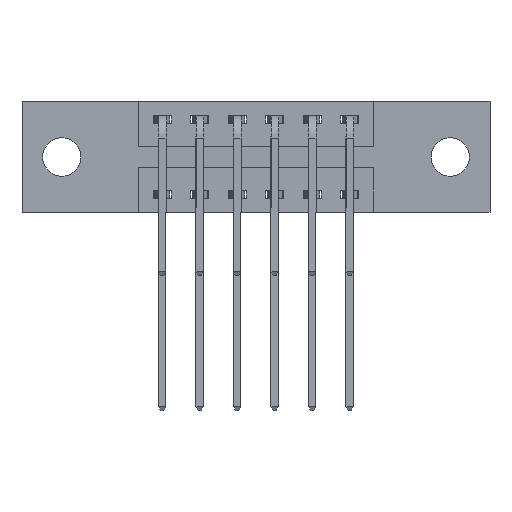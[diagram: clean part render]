
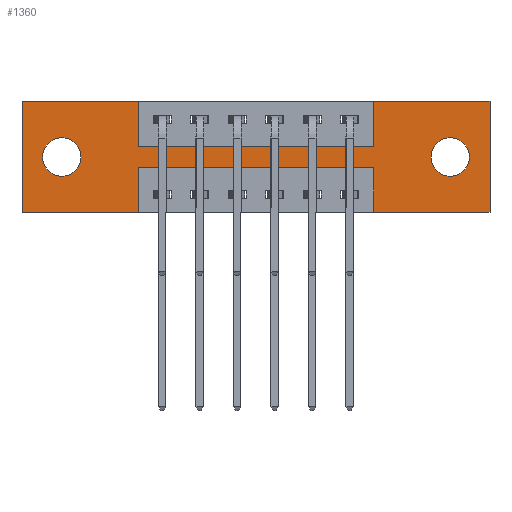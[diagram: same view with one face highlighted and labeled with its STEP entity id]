
A CAD part, front view. The second image highlights one B-rep face of the part: STEP entity #1360.
In plain terms, the highlighted planar face has unit normal (0, -1, 0).
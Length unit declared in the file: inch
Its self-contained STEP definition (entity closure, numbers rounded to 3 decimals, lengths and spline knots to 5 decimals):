
#8 = CARTESIAN_POINT ( 'NONE',  ( 1.56, 0., 0. ) ) ;
#78 = CARTESIAN_POINT ( 'NONE',  ( 0., 0., 0. ) ) ;
#110 = CARTESIAN_POINT ( 'NONE',  ( 0.3875, 0., -0.15 ) ) ;
#120 = LINE ( 'NONE', #2694, #4599 ) ;
#179 = CARTESIAN_POINT ( 'NONE',  ( 0.3875, 0., 0. ) ) ;
#503 = CARTESIAN_POINT ( 'NONE',  ( 0., 0., -0.37 ) ) ;
#523 = ORIENTED_EDGE ( 'NONE', *, *, #1006, .T. ) ;
#839 = DIRECTION ( 'NONE',  ( 0., 0., 1. ) ) ;
#906 = DIRECTION ( 'NONE',  ( 1., 0., 0. ) ) ;
#909 = EDGE_LOOP ( 'NONE', ( #4469, #9878 ) ) ;
#922 = VERTEX_POINT ( 'NONE', #8142 ) ;
#1006 = EDGE_CURVE ( 'NONE', #922, #10519, #6691, .T. ) ;
#1049 = LINE ( 'NONE', #110, #5203 ) ;
#1198 = EDGE_CURVE ( 'NONE', #1411, #8099, #6071, .T. ) ;
#1360 = ADVANCED_FACE ( 'NONE', ( #3206, #5055, #7134 ), #6268, .T. ) ;
#1411 = VERTEX_POINT ( 'NONE', #6201 ) ;
#1429 = DIRECTION ( 'NONE',  ( -1., 0., 0. ) ) ;
#1468 = DIRECTION ( 'NONE',  ( 1., 0., 0. ) ) ;
#1598 = EDGE_LOOP ( 'NONE', ( #10028, #1621, #8962, #8791, #6315, #3848, #6308, #6206, #7337, #6058, #9000, #7433 ) ) ;
#1621 = ORIENTED_EDGE ( 'NONE', *, *, #5158, .F. ) ;
#1800 = VERTEX_POINT ( 'NONE', #5182 ) ;
#1853 = LINE ( 'NONE', #2755, #8150 ) ;
#1967 = CARTESIAN_POINT ( 'NONE',  ( 1.1725, 0., 0. ) ) ;
#2053 = DIRECTION ( 'NONE',  ( 0., 1., 0. ) ) ;
#2152 = VECTOR ( 'NONE', #1429, 39.37008 ) ;
#2493 = CARTESIAN_POINT ( 'NONE',  ( 1.4275, 0., -0.249 ) ) ;
#2647 = CARTESIAN_POINT ( 'NONE',  ( 1.4275, 0., -0.185 ) ) ;
#2694 = CARTESIAN_POINT ( 'NONE',  ( 0.3875, 0., -0.37 ) ) ;
#2755 = CARTESIAN_POINT ( 'NONE',  ( 0., 0., 0. ) ) ;
#3206 = FACE_BOUND ( 'NONE', #909, .T. ) ;
#3214 = EDGE_LOOP ( 'NONE', ( #9630, #523 ) ) ;
#3297 = AXIS2_PLACEMENT_3D ( 'NONE', #7207, #4465, #5010 ) ;
#3348 = LINE ( 'NONE', #1967, #7286 ) ;
#3433 = CARTESIAN_POINT ( 'NONE',  ( 0., 0., -0.37 ) ) ;
#3558 = DIRECTION ( 'NONE',  ( 0., 0., -1. ) ) ;
#3589 = VECTOR ( 'NONE', #5316, 39.37008 ) ;
#3848 = ORIENTED_EDGE ( 'NONE', *, *, #1198, .F. ) ;
#4050 = VERTEX_POINT ( 'NONE', #2493 ) ;
#4059 = VERTEX_POINT ( 'NONE', #3433 ) ;
#4079 = LINE ( 'NONE', #7612, #10232 ) ;
#4196 = VERTEX_POINT ( 'NONE', #7452 ) ;
#4286 = EDGE_CURVE ( 'NONE', #4059, #4196, #1853, .T. ) ;
#4334 = LINE ( 'NONE', #9366, #6192 ) ;
#4375 = EDGE_CURVE ( 'NONE', #8099, #6801, #7669, .T. ) ;
#4419 = DIRECTION ( 'NONE',  ( 0., 0., 1. ) ) ;
#4465 = DIRECTION ( 'NONE',  ( 0., 1., 0. ) ) ;
#4469 = ORIENTED_EDGE ( 'NONE', *, *, #4899, .T. ) ;
#4475 = EDGE_CURVE ( 'NONE', #4050, #8294, #6928, .T. ) ;
#4529 = CARTESIAN_POINT ( 'NONE',  ( 0.3875, 0., -0.22 ) ) ;
#4531 = EDGE_CURVE ( 'NONE', #6801, #1800, #4334, .T. ) ;
#4570 = DIRECTION ( 'NONE',  ( 0., 0., 1. ) ) ;
#4599 = VECTOR ( 'NONE', #5973, 39.37008 ) ;
#4742 = EDGE_CURVE ( 'NONE', #8992, #4059, #8492, .T. ) ;
#4782 = LINE ( 'NONE', #78, #8660 ) ;
#4784 = DIRECTION ( 'NONE',  ( 0., 0., -1. ) ) ;
#4899 = EDGE_CURVE ( 'NONE', #8294, #4050, #5324, .T. ) ;
#4996 = EDGE_CURVE ( 'NONE', #8568, #8992, #120, .T. ) ;
#5010 = DIRECTION ( 'NONE',  ( 0., 0., 1. ) ) ;
#5011 = AXIS2_PLACEMENT_3D ( 'NONE', #2647, #8249, #3558 ) ;
#5014 = EDGE_CURVE ( 'NONE', #10519, #922, #6427, .T. ) ;
#5055 = FACE_BOUND ( 'NONE', #3214, .T. ) ;
#5075 = EDGE_CURVE ( 'NONE', #1800, #9002, #4079, .T. ) ;
#5158 = EDGE_CURVE ( 'NONE', #9002, #8568, #8027, .T. ) ;
#5182 = CARTESIAN_POINT ( 'NONE',  ( 1.1725, 0., -0.37 ) ) ;
#5191 = EDGE_CURVE ( 'NONE', #6055, #8552, #1049, .T. ) ;
#5193 = EDGE_CURVE ( 'NONE', #8552, #1411, #3348, .T. ) ;
#5203 = VECTOR ( 'NONE', #6924, 39.37008 ) ;
#5217 = CARTESIAN_POINT ( 'NONE',  ( 0.1325, 0., -0.185 ) ) ;
#5219 = CARTESIAN_POINT ( 'NONE',  ( 1.1725, 0., -0.22 ) ) ;
#5316 = DIRECTION ( 'NONE',  ( -1., 0., 0. ) ) ;
#5322 = EDGE_CURVE ( 'NONE', #9239, #6055, #8357, .T. ) ;
#5323 = DIRECTION ( 'NONE',  ( 0., 0., -1. ) ) ;
#5324 = CIRCLE ( 'NONE', #5011, 0.064 ) ;
#5590 = VECTOR ( 'NONE', #5323, 39.37008 ) ;
#5720 = CARTESIAN_POINT ( 'NONE',  ( 0.1325, 0., -0.121 ) ) ;
#5768 = CARTESIAN_POINT ( 'NONE',  ( 0.3875, 0., -0.22 ) ) ;
#5826 = VECTOR ( 'NONE', #1468, 39.37008 ) ;
#5973 = DIRECTION ( 'NONE',  ( 0., 0., -1. ) ) ;
#6006 = DIRECTION ( 'NONE',  ( 0., 0., 1. ) ) ;
#6055 = VERTEX_POINT ( 'NONE', #6158 ) ;
#6056 = AXIS2_PLACEMENT_3D ( 'NONE', #5217, #10553, #6006 ) ;
#6058 = ORIENTED_EDGE ( 'NONE', *, *, #9107, .F. ) ;
#6071 = LINE ( 'NONE', #10139, #5826 ) ;
#6158 = CARTESIAN_POINT ( 'NONE',  ( 0.3875, 0., -0.15 ) ) ;
#6192 = VECTOR ( 'NONE', #10109, 39.37008 ) ;
#6201 = CARTESIAN_POINT ( 'NONE',  ( 1.1725, 0., 0. ) ) ;
#6206 = ORIENTED_EDGE ( 'NONE', *, *, #5191, .F. ) ;
#6268 = PLANE ( 'NONE',  #10288 ) ;
#6308 = ORIENTED_EDGE ( 'NONE', *, *, #5193, .F. ) ;
#6315 = ORIENTED_EDGE ( 'NONE', *, *, #4375, .F. ) ;
#6427 = CIRCLE ( 'NONE', #6056, 0.064 ) ;
#6691 = CIRCLE ( 'NONE', #3297, 0.064 ) ;
#6801 = VERTEX_POINT ( 'NONE', #8296 ) ;
#6924 = DIRECTION ( 'NONE',  ( 1., 0., 0. ) ) ;
#6928 = CIRCLE ( 'NONE', #8830, 0.064 ) ;
#6998 = CARTESIAN_POINT ( 'NONE',  ( 1.4275, 0., -0.185 ) ) ;
#7134 = FACE_OUTER_BOUND ( 'NONE', #1598, .T. ) ;
#7207 = CARTESIAN_POINT ( 'NONE',  ( 0.1325, 0., -0.185 ) ) ;
#7286 = VECTOR ( 'NONE', #4570, 39.37008 ) ;
#7337 = ORIENTED_EDGE ( 'NONE', *, *, #5322, .F. ) ;
#7342 = CARTESIAN_POINT ( 'NONE',  ( 0., 0., -0.37 ) ) ;
#7433 = ORIENTED_EDGE ( 'NONE', *, *, #4742, .F. ) ;
#7452 = CARTESIAN_POINT ( 'NONE',  ( 0., 0., 0. ) ) ;
#7612 = CARTESIAN_POINT ( 'NONE',  ( 1.1725, 0., -0.37 ) ) ;
#7669 = LINE ( 'NONE', #8, #5590 ) ;
#7788 = DIRECTION ( 'NONE',  ( 0., 0., -1. ) ) ;
#7800 = DIRECTION ( 'NONE',  ( 0., 0., -1. ) ) ;
#7801 = CARTESIAN_POINT ( 'NONE',  ( 1.56, 0., 0. ) ) ;
#8027 = LINE ( 'NONE', #4529, #3589 ) ;
#8099 = VERTEX_POINT ( 'NONE', #7801 ) ;
#8131 = VECTOR ( 'NONE', #7788, 39.37008 ) ;
#8142 = CARTESIAN_POINT ( 'NONE',  ( 0.1325, 0., -0.249 ) ) ;
#8150 = VECTOR ( 'NONE', #4419, 39.37008 ) ;
#8249 = DIRECTION ( 'NONE',  ( 0., 1., 0. ) ) ;
#8294 = VERTEX_POINT ( 'NONE', #10182 ) ;
#8296 = CARTESIAN_POINT ( 'NONE',  ( 1.56, 0., -0.37 ) ) ;
#8357 = LINE ( 'NONE', #10035, #8131 ) ;
#8492 = LINE ( 'NONE', #503, #2152 ) ;
#8552 = VERTEX_POINT ( 'NONE', #9619 ) ;
#8568 = VERTEX_POINT ( 'NONE', #5768 ) ;
#8660 = VECTOR ( 'NONE', #906, 39.37008 ) ;
#8791 = ORIENTED_EDGE ( 'NONE', *, *, #4531, .F. ) ;
#8830 = AXIS2_PLACEMENT_3D ( 'NONE', #6998, #2053, #7800 ) ;
#8962 = ORIENTED_EDGE ( 'NONE', *, *, #5075, .F. ) ;
#8992 = VERTEX_POINT ( 'NONE', #10555 ) ;
#9000 = ORIENTED_EDGE ( 'NONE', *, *, #4286, .F. ) ;
#9002 = VERTEX_POINT ( 'NONE', #5219 ) ;
#9107 = EDGE_CURVE ( 'NONE', #4196, #9239, #4782, .T. ) ;
#9239 = VERTEX_POINT ( 'NONE', #179 ) ;
#9366 = CARTESIAN_POINT ( 'NONE',  ( 0., 0., -0.37 ) ) ;
#9619 = CARTESIAN_POINT ( 'NONE',  ( 1.1725, 0., -0.15 ) ) ;
#9630 = ORIENTED_EDGE ( 'NONE', *, *, #5014, .T. ) ;
#9708 = DIRECTION ( 'NONE',  ( 0., -1., 0. ) ) ;
#9878 = ORIENTED_EDGE ( 'NONE', *, *, #4475, .T. ) ;
#10028 = ORIENTED_EDGE ( 'NONE', *, *, #4996, .F. ) ;
#10035 = CARTESIAN_POINT ( 'NONE',  ( 0.3875, 0., 0. ) ) ;
#10109 = DIRECTION ( 'NONE',  ( -1., 0., 0. ) ) ;
#10139 = CARTESIAN_POINT ( 'NONE',  ( 0., 0., 0. ) ) ;
#10182 = CARTESIAN_POINT ( 'NONE',  ( 1.4275, 0., -0.121 ) ) ;
#10232 = VECTOR ( 'NONE', #839, 39.37008 ) ;
#10288 = AXIS2_PLACEMENT_3D ( 'NONE', #7342, #9708, #4784 ) ;
#10519 = VERTEX_POINT ( 'NONE', #5720 ) ;
#10553 = DIRECTION ( 'NONE',  ( 0., 1., 0. ) ) ;
#10555 = CARTESIAN_POINT ( 'NONE',  ( 0.3875, 0., -0.37 ) ) ;
